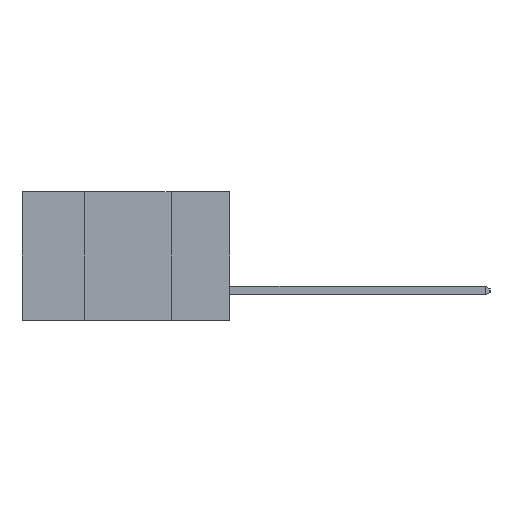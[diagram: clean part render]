
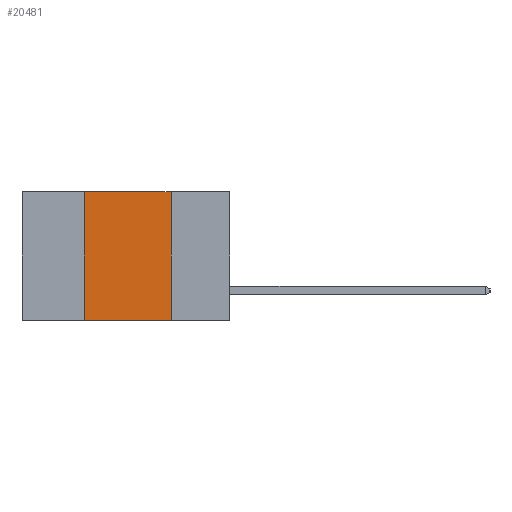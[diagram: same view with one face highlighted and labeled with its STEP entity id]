
A CAD part, left-side view. The second image highlights one B-rep face of the part: STEP entity #20481.
In plain terms, the highlighted planar face has unit normal (-1, 0, 0).
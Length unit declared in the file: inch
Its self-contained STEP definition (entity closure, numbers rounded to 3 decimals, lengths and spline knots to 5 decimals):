
#195 = DIRECTION ( 'NONE',  ( 0., 0., -1. ) ) ;
#857 = DIRECTION ( 'NONE',  ( 0., -1., 0. ) ) ;
#1014 = EDGE_LOOP ( 'NONE', ( #11474, #5360, #1067, #11970 ) ) ;
#1067 = ORIENTED_EDGE ( 'NONE', *, *, #27214, .F. ) ;
#2127 = CARTESIAN_POINT ( 'NONE',  ( 0., 0.17, 0. ) ) ;
#2555 = EDGE_CURVE ( 'NONE', #2970, #26282, #25577, .T. ) ;
#2699 = AXIS2_PLACEMENT_3D ( 'NONE', #10691, #12834, #195 ) ;
#2970 = VERTEX_POINT ( 'NONE', #2127 ) ;
#4342 = VERTEX_POINT ( 'NONE', #21733 ) ;
#5360 = ORIENTED_EDGE ( 'NONE', *, *, #26544, .F. ) ;
#5625 = CARTESIAN_POINT ( 'NONE',  ( 0., 0.42, 0. ) ) ;
#5785 = DIRECTION ( 'NONE',  ( 0., 0., -1. ) ) ;
#8178 = CARTESIAN_POINT ( 'NONE',  ( 0., 0.17, 0. ) ) ;
#8564 = PLANE ( 'NONE',  #2699 ) ;
#9515 = VECTOR ( 'NONE', #20698, 39.37008 ) ;
#9661 = FACE_OUTER_BOUND ( 'NONE', #1014, .T. ) ;
#10202 = VERTEX_POINT ( 'NONE', #5625 ) ;
#10691 = CARTESIAN_POINT ( 'NONE',  ( 0., 0.6, 0. ) ) ;
#10797 = VECTOR ( 'NONE', #15561, 39.37008 ) ;
#11363 = CARTESIAN_POINT ( 'NONE',  ( 0., 0.6, 0. ) ) ;
#11474 = ORIENTED_EDGE ( 'NONE', *, *, #2555, .F. ) ;
#11970 = ORIENTED_EDGE ( 'NONE', *, *, #22980, .T. ) ;
#12834 = DIRECTION ( 'NONE',  ( 1., 0., 0. ) ) ;
#15561 = DIRECTION ( 'NONE',  ( 0., -1., 0. ) ) ;
#16498 = LINE ( 'NONE', #23939, #10797 ) ;
#18054 = CARTESIAN_POINT ( 'NONE',  ( 0., 0.42, 0. ) ) ;
#18849 = CARTESIAN_POINT ( 'NONE',  ( 0., 0.17, -0.37 ) ) ;
#20481 = ADVANCED_FACE ( 'NONE', ( #9661 ), #8564, .F. ) ;
#20698 = DIRECTION ( 'NONE',  ( 0., 0., 1. ) ) ;
#21733 = CARTESIAN_POINT ( 'NONE',  ( 0., 0.42, -0.37 ) ) ;
#22574 = VECTOR ( 'NONE', #857, 39.37008 ) ;
#22980 = EDGE_CURVE ( 'NONE', #4342, #26282, #16498, .T. ) ;
#23234 = LINE ( 'NONE', #11363, #22574 ) ;
#23939 = CARTESIAN_POINT ( 'NONE',  ( 0., 0.6, -0.37 ) ) ;
#24247 = VECTOR ( 'NONE', #5785, 39.37008 ) ;
#25577 = LINE ( 'NONE', #8178, #24247 ) ;
#26282 = VERTEX_POINT ( 'NONE', #18849 ) ;
#26495 = LINE ( 'NONE', #18054, #9515 ) ;
#26544 = EDGE_CURVE ( 'NONE', #10202, #2970, #23234, .T. ) ;
#27214 = EDGE_CURVE ( 'NONE', #4342, #10202, #26495, .T. ) ;
